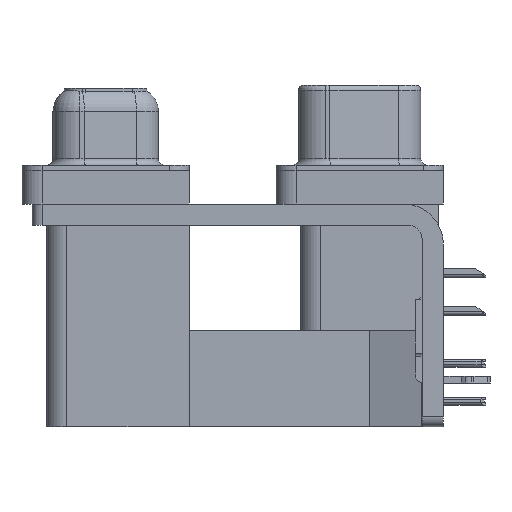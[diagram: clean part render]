
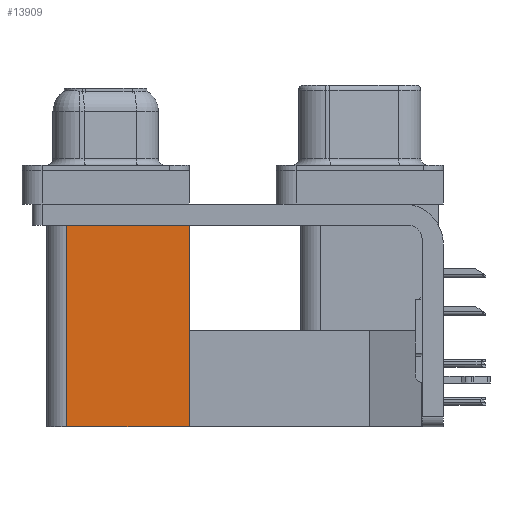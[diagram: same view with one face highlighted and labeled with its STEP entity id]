
A CAD part, left-side view. The second image highlights one B-rep face of the part: STEP entity #13909.
In plain terms, the highlighted planar face has unit normal (-1, 0, 0).
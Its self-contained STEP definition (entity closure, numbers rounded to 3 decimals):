
#351 = LINE ( 'NONE', #8882, #19439 ) ;
#1149 = AXIS2_PLACEMENT_3D ( 'NONE', #17795, #33256, #33068 ) ;
#2477 = VERTEX_POINT ( 'NONE', #37108 ) ;
#2533 = CARTESIAN_POINT ( 'NONE',  ( 3.79, 12.775, -2.5 ) ) ;
#6911 = EDGE_CURVE ( 'NONE', #35626, #15874, #351, .T. ) ;
#8882 = CARTESIAN_POINT ( 'NONE',  ( 3.79, 21.975, -19.2 ) ) ;
#9878 = DIRECTION ( 'NONE',  ( 0., 1., 0. ) ) ;
#10585 = VECTOR ( 'NONE', #36033, 1000. ) ;
#13804 = CARTESIAN_POINT ( 'NONE',  ( 3.79, 21.975, -19.2 ) ) ;
#13909 = ADVANCED_FACE ( 'NONE', ( #38396 ), #29716, .F. ) ;
#15874 = VERTEX_POINT ( 'NONE', #18055 ) ;
#16519 = VECTOR ( 'NONE', #9878, 1000. ) ;
#16746 = ORIENTED_EDGE ( 'NONE', *, *, #27432, .F. ) ;
#16996 = DIRECTION ( 'NONE',  ( 0., 1., 0. ) ) ;
#17571 = CARTESIAN_POINT ( 'NONE',  ( 3.79, 12.775, -2.5 ) ) ;
#17795 = CARTESIAN_POINT ( 'NONE',  ( 3.79, 12.775, -19.2 ) ) ;
#18055 = CARTESIAN_POINT ( 'NONE',  ( 3.79, 21.975, -2.5 ) ) ;
#19439 = VECTOR ( 'NONE', #30674, 1000. ) ;
#22412 = VERTEX_POINT ( 'NONE', #17571 ) ;
#27121 = LINE ( 'NONE', #32473, #10585 ) ;
#27432 = EDGE_CURVE ( 'NONE', #2477, #35626, #27924, .T. ) ;
#27924 = LINE ( 'NONE', #33863, #16519 ) ;
#28100 = ORIENTED_EDGE ( 'NONE', *, *, #6911, .F. ) ;
#29167 = EDGE_CURVE ( 'NONE', #2477, #22412, #27121, .T. ) ;
#29716 = PLANE ( 'NONE',  #1149 ) ;
#30674 = DIRECTION ( 'NONE',  ( 0., 0., 1. ) ) ;
#30936 = ORIENTED_EDGE ( 'NONE', *, *, #38030, .T. ) ;
#31387 = VECTOR ( 'NONE', #16996, 1000. ) ;
#32050 = LINE ( 'NONE', #2533, #31387 ) ;
#32473 = CARTESIAN_POINT ( 'NONE',  ( 3.79, 12.775, -19.2 ) ) ;
#33068 = DIRECTION ( 'NONE',  ( 0., 1., 0. ) ) ;
#33256 = DIRECTION ( 'NONE',  ( 1., 0., 0. ) ) ;
#33863 = CARTESIAN_POINT ( 'NONE',  ( 3.79, 12.775, -19.2 ) ) ;
#35626 = VERTEX_POINT ( 'NONE', #13804 ) ;
#36033 = DIRECTION ( 'NONE',  ( 0., 0., 1. ) ) ;
#36755 = EDGE_LOOP ( 'NONE', ( #30936, #28100, #16746, #38370 ) ) ;
#37108 = CARTESIAN_POINT ( 'NONE',  ( 3.79, 12.775, -19.2 ) ) ;
#38030 = EDGE_CURVE ( 'NONE', #22412, #15874, #32050, .T. ) ;
#38370 = ORIENTED_EDGE ( 'NONE', *, *, #29167, .T. ) ;
#38396 = FACE_OUTER_BOUND ( 'NONE', #36755, .T. ) ;
